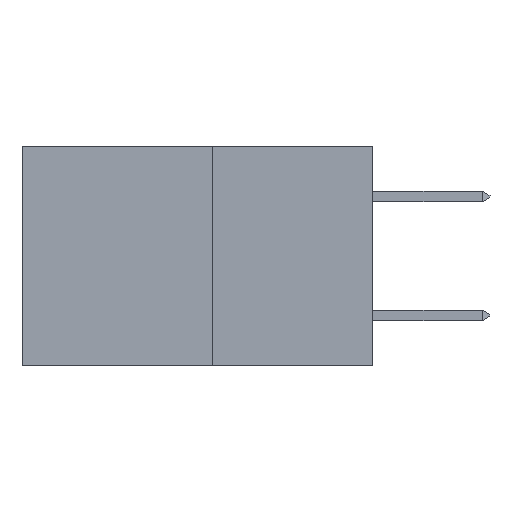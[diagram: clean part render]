
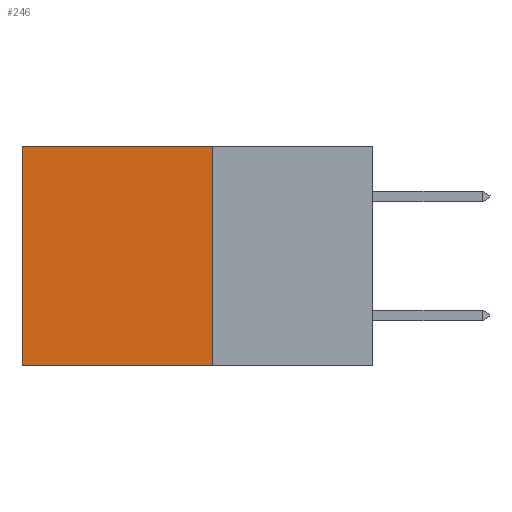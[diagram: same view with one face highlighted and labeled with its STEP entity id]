
A CAD part, left-side view. The second image highlights one B-rep face of the part: STEP entity #246.
In plain terms, the highlighted planar face has unit normal (-1, 0, 0).
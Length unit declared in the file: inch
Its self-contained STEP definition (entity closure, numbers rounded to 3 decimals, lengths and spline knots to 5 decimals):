
#246 = ADVANCED_FACE ( 'NONE', ( #2231 ), #4860, .F. ) ;
#1524 = VERTEX_POINT ( 'NONE', #3403 ) ;
#1748 = EDGE_CURVE ( 'NONE', #4841, #5011, #12699, .T. ) ;
#1897 = VECTOR ( 'NONE', #6455, 39.37008 ) ;
#2009 = VERTEX_POINT ( 'NONE', #4235 ) ;
#2231 = FACE_OUTER_BOUND ( 'NONE', #5830, .T. ) ;
#2956 = DIRECTION ( 'NONE',  ( 0., 0., -1. ) ) ;
#3364 = LINE ( 'NONE', #4190, #8350 ) ;
#3403 = CARTESIAN_POINT ( 'NONE',  ( 0.277, 0.59, -0.37 ) ) ;
#3978 = ORIENTED_EDGE ( 'NONE', *, *, #10631, .F. ) ;
#4103 = VECTOR ( 'NONE', #7064, 39.37008 ) ;
#4190 = CARTESIAN_POINT ( 'NONE',  ( 0.277, 0.27, -0.37 ) ) ;
#4224 = DIRECTION ( 'NONE',  ( 0., 0., -1. ) ) ;
#4235 = CARTESIAN_POINT ( 'NONE',  ( 0.277, 0.27, -0.37 ) ) ;
#4439 = DIRECTION ( 'NONE',  ( 1., 0., 0. ) ) ;
#4841 = VERTEX_POINT ( 'NONE', #12095 ) ;
#4860 = PLANE ( 'NONE',  #8377 ) ;
#4938 = VECTOR ( 'NONE', #4224, 39.37008 ) ;
#4998 = ORIENTED_EDGE ( 'NONE', *, *, #1748, .T. ) ;
#5011 = VERTEX_POINT ( 'NONE', #11165 ) ;
#5181 = DIRECTION ( 'NONE',  ( 0., 1., 0. ) ) ;
#5830 = EDGE_LOOP ( 'NONE', ( #9299, #3978, #11442, #4998 ) ) ;
#6056 = CARTESIAN_POINT ( 'NONE',  ( 0.277, 0.27, -0.37 ) ) ;
#6238 = CARTESIAN_POINT ( 'NONE',  ( 0.277, 0.59, -0.37 ) ) ;
#6455 = DIRECTION ( 'NONE',  ( 0., 1., 0. ) ) ;
#6458 = CARTESIAN_POINT ( 'NONE',  ( 0.277, 0.27, 0. ) ) ;
#6775 = LINE ( 'NONE', #6056, #4103 ) ;
#7013 = EDGE_CURVE ( 'NONE', #5011, #1524, #12552, .T. ) ;
#7064 = DIRECTION ( 'NONE',  ( 0., 0., -1. ) ) ;
#8350 = VECTOR ( 'NONE', #5181, 39.37008 ) ;
#8377 = AXIS2_PLACEMENT_3D ( 'NONE', #8561, #4439, #2956 ) ;
#8561 = CARTESIAN_POINT ( 'NONE',  ( 0.277, 0.27, -0.37 ) ) ;
#9299 = ORIENTED_EDGE ( 'NONE', *, *, #7013, .T. ) ;
#10631 = EDGE_CURVE ( 'NONE', #2009, #1524, #3364, .T. ) ;
#11165 = CARTESIAN_POINT ( 'NONE',  ( 0.277, 0.59, 0. ) ) ;
#11281 = EDGE_CURVE ( 'NONE', #4841, #2009, #6775, .T. ) ;
#11442 = ORIENTED_EDGE ( 'NONE', *, *, #11281, .F. ) ;
#12095 = CARTESIAN_POINT ( 'NONE',  ( 0.277, 0.27, 0. ) ) ;
#12552 = LINE ( 'NONE', #6238, #4938 ) ;
#12699 = LINE ( 'NONE', #6458, #1897 ) ;
